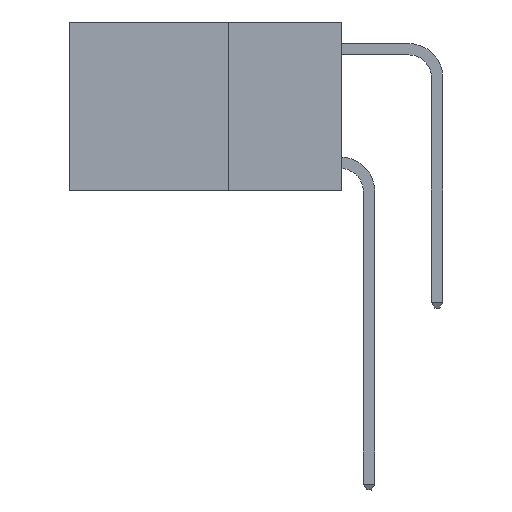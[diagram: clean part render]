
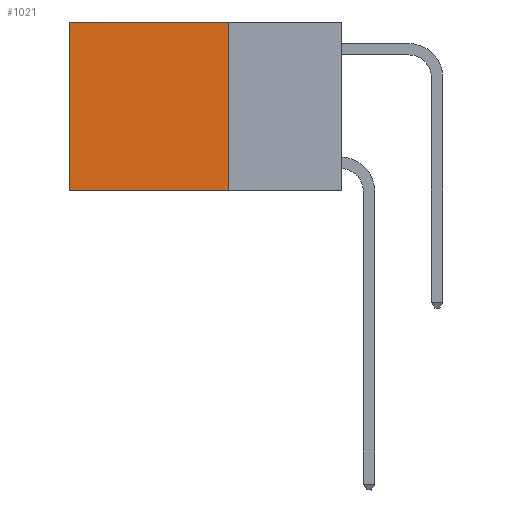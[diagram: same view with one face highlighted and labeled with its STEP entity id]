
A CAD part, left-side view. The second image highlights one B-rep face of the part: STEP entity #1021.
In plain terms, the highlighted planar face has unit normal (-1, 0, 0).
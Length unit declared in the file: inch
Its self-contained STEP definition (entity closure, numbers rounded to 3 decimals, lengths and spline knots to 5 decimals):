
#109 = VERTEX_POINT ( 'NONE', #10695 ) ;
#1021 = ADVANCED_FACE ( 'NONE', ( #12157 ), #2221, .F. ) ;
#1680 = LINE ( 'NONE', #1865, #6569 ) ;
#1865 = CARTESIAN_POINT ( 'NONE',  ( 0.2625, 0.25, 0. ) ) ;
#2221 = PLANE ( 'NONE',  #10456 ) ;
#2351 = CARTESIAN_POINT ( 'NONE',  ( 0.2625, 0.6, 0. ) ) ;
#2418 = EDGE_CURVE ( 'NONE', #2658, #109, #3225, .T. ) ;
#2658 = VERTEX_POINT ( 'NONE', #8882 ) ;
#2677 = DIRECTION ( 'NONE',  ( 0., 1., 0. ) ) ;
#2813 = DIRECTION ( 'NONE',  ( 0., 1., 0. ) ) ;
#2877 = CARTESIAN_POINT ( 'NONE',  ( 0.2625, 0.25, -0.37 ) ) ;
#2901 = VECTOR ( 'NONE', #8035, 39.37008 ) ;
#3225 = LINE ( 'NONE', #2877, #8207 ) ;
#3314 = EDGE_CURVE ( 'NONE', #12079, #2658, #10998, .T. ) ;
#3406 = DIRECTION ( 'NONE',  ( 1., 0., 0. ) ) ;
#5283 = DIRECTION ( 'NONE',  ( 0., 0., -1. ) ) ;
#5629 = VECTOR ( 'NONE', #5283, 39.37008 ) ;
#6295 = ORIENTED_EDGE ( 'NONE', *, *, #3314, .F. ) ;
#6371 = CARTESIAN_POINT ( 'NONE',  ( 0.2625, 0.25, 0. ) ) ;
#6569 = VECTOR ( 'NONE', #2813, 39.37008 ) ;
#7039 = CARTESIAN_POINT ( 'NONE',  ( 0.2625, 0.25, 0. ) ) ;
#7064 = VERTEX_POINT ( 'NONE', #9813 ) ;
#8035 = DIRECTION ( 'NONE',  ( 0., 0., -1. ) ) ;
#8207 = VECTOR ( 'NONE', #2677, 39.37008 ) ;
#8616 = ORIENTED_EDGE ( 'NONE', *, *, #10891, .T. ) ;
#8882 = CARTESIAN_POINT ( 'NONE',  ( 0.2625, 0.25, -0.37 ) ) ;
#8902 = ORIENTED_EDGE ( 'NONE', *, *, #2418, .F. ) ;
#9009 = EDGE_LOOP ( 'NONE', ( #8616, #8902, #6295, #11715 ) ) ;
#9450 = CARTESIAN_POINT ( 'NONE',  ( 0.2625, 0.25, 0. ) ) ;
#9813 = CARTESIAN_POINT ( 'NONE',  ( 0.2625, 0.6, 0. ) ) ;
#9953 = DIRECTION ( 'NONE',  ( 0., 0., -1. ) ) ;
#10456 = AXIS2_PLACEMENT_3D ( 'NONE', #9450, #3406, #9953 ) ;
#10695 = CARTESIAN_POINT ( 'NONE',  ( 0.2625, 0.6, -0.37 ) ) ;
#10891 = EDGE_CURVE ( 'NONE', #7064, #109, #11096, .T. ) ;
#10998 = LINE ( 'NONE', #7039, #2901 ) ;
#11096 = LINE ( 'NONE', #2351, #5629 ) ;
#11278 = EDGE_CURVE ( 'NONE', #12079, #7064, #1680, .T. ) ;
#11715 = ORIENTED_EDGE ( 'NONE', *, *, #11278, .T. ) ;
#12079 = VERTEX_POINT ( 'NONE', #6371 ) ;
#12157 = FACE_OUTER_BOUND ( 'NONE', #9009, .T. ) ;
